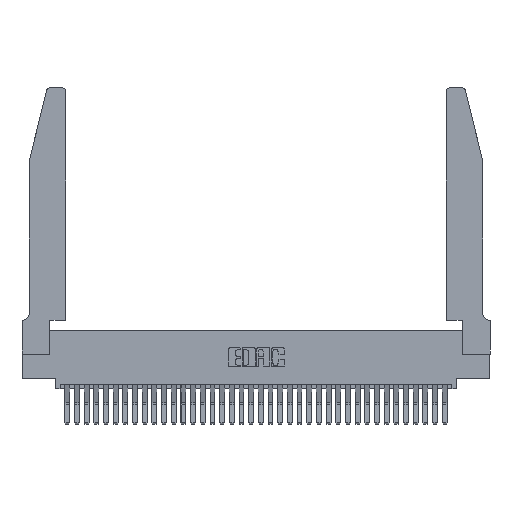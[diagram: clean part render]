
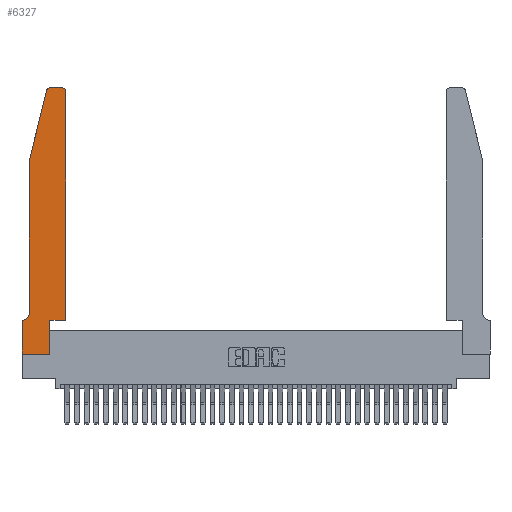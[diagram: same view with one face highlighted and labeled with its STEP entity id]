
A CAD part, top view. The second image highlights one B-rep face of the part: STEP entity #6327.
In plain terms, the highlighted planar face has unit normal (0, 0, 1).
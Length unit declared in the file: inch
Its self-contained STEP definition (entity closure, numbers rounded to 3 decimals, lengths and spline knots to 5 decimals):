
#99 = LINE ( 'NONE', #27117, #14691 ) ;
#202 = DIRECTION ( 'NONE',  ( -1., 0., 0. ) ) ;
#450 = CARTESIAN_POINT ( 'NONE',  ( 0.4205, 2.72, 0.37 ) ) ;
#1453 = DIRECTION ( 'NONE',  ( 0., 1., 0. ) ) ;
#1481 = ORIENTED_EDGE ( 'NONE', *, *, #2511, .T. ) ;
#1762 = CARTESIAN_POINT ( 'NONE',  ( 0.2605, 2.75, 0.37 ) ) ;
#2511 = EDGE_CURVE ( 'NONE', #35598, #21284, #27533, .T. ) ;
#2516 = VERTEX_POINT ( 'NONE', #13177 ) ;
#2844 = AXIS2_PLACEMENT_3D ( 'NONE', #29377, #12700, #32178 ) ;
#3141 = VECTOR ( 'NONE', #26268, 39.37008 ) ;
#3402 = DIRECTION ( 'NONE',  ( 1., 0., 0. ) ) ;
#3568 = CARTESIAN_POINT ( 'NONE',  ( 0.0755, 0.35, 0.37 ) ) ;
#3908 = CARTESIAN_POINT ( 'NONE',  ( 0.284, 2.75, 0.37 ) ) ;
#4074 = ORIENTED_EDGE ( 'NONE', *, *, #31906, .T. ) ;
#4113 = ORIENTED_EDGE ( 'NONE', *, *, #31915, .T. ) ;
#4151 = ORIENTED_EDGE ( 'NONE', *, *, #13359, .T. ) ;
#4364 = VERTEX_POINT ( 'NONE', #22695 ) ;
#4402 = CARTESIAN_POINT ( 'NONE',  ( 0.2865, 0.35, 0.37 ) ) ;
#4698 = CARTESIAN_POINT ( 'NONE',  ( 0., 0., 0.37 ) ) ;
#4884 = VERTEX_POINT ( 'NONE', #19773 ) ;
#4965 = VECTOR ( 'NONE', #1453, 39.37008 ) ;
#5477 = PLANE ( 'NONE',  #13334 ) ;
#5591 = DIRECTION ( 'NONE',  ( 1., 0., 0. ) ) ;
#6061 = EDGE_CURVE ( 'NONE', #27158, #4364, #34232, .T. ) ;
#6327 = ADVANCED_FACE ( 'NONE', ( #26391 ), #5477, .T. ) ;
#6561 = LINE ( 'NONE', #23788, #27309 ) ;
#6644 = EDGE_CURVE ( 'NONE', #10097, #32319, #24177, .T. ) ;
#7117 = CARTESIAN_POINT ( 'NONE',  ( 0., 0., 0.37 ) ) ;
#7408 = DIRECTION ( 'NONE',  ( 0., -1., 0. ) ) ;
#7522 = DIRECTION ( 'NONE',  ( -1., 0., 0. ) ) ;
#7606 = EDGE_LOOP ( 'NONE', ( #29742, #34257, #24436, #26052, #4074, #9270, #14604, #16992, #1481, #4113, #4151, #17957 ) ) ;
#7852 = CIRCLE ( 'NONE', #8065, 0.07 ) ;
#8065 = AXIS2_PLACEMENT_3D ( 'NONE', #34139, #17550, #202 ) ;
#8602 = AXIS2_PLACEMENT_3D ( 'NONE', #450, #20549, #3402 ) ;
#8672 = CIRCLE ( 'NONE', #8602, 0.03 ) ;
#8950 = VECTOR ( 'NONE', #27343, 39.37008 ) ;
#9270 = ORIENTED_EDGE ( 'NONE', *, *, #16638, .T. ) ;
#9965 = EDGE_CURVE ( 'NONE', #4884, #2516, #8672, .T. ) ;
#10097 = VERTEX_POINT ( 'NONE', #3908 ) ;
#11513 = CARTESIAN_POINT ( 'NONE',  ( 0.0755, 0.42, 0.37 ) ) ;
#11669 = EDGE_CURVE ( 'NONE', #2516, #10097, #36123, .T. ) ;
#12108 = CARTESIAN_POINT ( 'NONE',  ( 0.0755, 2., 0.37 ) ) ;
#12646 = CARTESIAN_POINT ( 'NONE',  ( 0.0755, 2., 0.37 ) ) ;
#12700 = DIRECTION ( 'NONE',  ( 0., 0., 1. ) ) ;
#13177 = CARTESIAN_POINT ( 'NONE',  ( 0.4205, 2.75, 0.37 ) ) ;
#13334 = AXIS2_PLACEMENT_3D ( 'NONE', #17090, #22622, #5591 ) ;
#13359 = EDGE_CURVE ( 'NONE', #24913, #4884, #6561, .T. ) ;
#13776 = CARTESIAN_POINT ( 'NONE',  ( 0.4505, 0.35, 0.37 ) ) ;
#14604 = ORIENTED_EDGE ( 'NONE', *, *, #6061, .T. ) ;
#14691 = VECTOR ( 'NONE', #7408, 39.37008 ) ;
#14724 = DIRECTION ( 'NONE',  ( 1., 0., 0. ) ) ;
#14790 = EDGE_CURVE ( 'NONE', #24642, #27037, #99, .T. ) ;
#14854 = VECTOR ( 'NONE', #7522, 39.37008 ) ;
#16638 = EDGE_CURVE ( 'NONE', #18704, #27158, #18467, .T. ) ;
#16992 = ORIENTED_EDGE ( 'NONE', *, *, #27493, .T. ) ;
#17090 = CARTESIAN_POINT ( 'NONE',  ( 0., 0.35, 0.37 ) ) ;
#17550 = DIRECTION ( 'NONE',  ( 0., 0., -1. ) ) ;
#17957 = ORIENTED_EDGE ( 'NONE', *, *, #9965, .T. ) ;
#18467 = LINE ( 'NONE', #3568, #3141 ) ;
#18704 = VERTEX_POINT ( 'NONE', #28279 ) ;
#19773 = CARTESIAN_POINT ( 'NONE',  ( 0.4505, 2.72, 0.37 ) ) ;
#20549 = DIRECTION ( 'NONE',  ( 0., 0., 1. ) ) ;
#21284 = VERTEX_POINT ( 'NONE', #22492 ) ;
#22060 = VECTOR ( 'NONE', #34887, 39.37008 ) ;
#22492 = CARTESIAN_POINT ( 'NONE',  ( 0.2865, 0.35, 0.37 ) ) ;
#22622 = DIRECTION ( 'NONE',  ( 0., 0., 1. ) ) ;
#22695 = CARTESIAN_POINT ( 'NONE',  ( 0., 0., 0.37 ) ) ;
#23493 = CARTESIAN_POINT ( 'NONE',  ( 0.2865, 0., 0.37 ) ) ;
#23788 = CARTESIAN_POINT ( 'NONE',  ( 0.4505, 0.35, 0.37 ) ) ;
#24177 = CIRCLE ( 'NONE', #2844, 0.03 ) ;
#24436 = ORIENTED_EDGE ( 'NONE', *, *, #31425, .T. ) ;
#24631 = LINE ( 'NONE', #12108, #22060 ) ;
#24642 = VERTEX_POINT ( 'NONE', #12646 ) ;
#24913 = VERTEX_POINT ( 'NONE', #13776 ) ;
#26052 = ORIENTED_EDGE ( 'NONE', *, *, #14790, .T. ) ;
#26268 = DIRECTION ( 'NONE',  ( -1., 0., 0. ) ) ;
#26391 = FACE_OUTER_BOUND ( 'NONE', #7606, .T. ) ;
#26604 = DIRECTION ( 'NONE',  ( 0., 1., 0. ) ) ;
#26848 = VECTOR ( 'NONE', #32432, 39.37008 ) ;
#27037 = VERTEX_POINT ( 'NONE', #11513 ) ;
#27117 = CARTESIAN_POINT ( 'NONE',  ( 0.0755, 2., 0.37 ) ) ;
#27158 = VERTEX_POINT ( 'NONE', #34287 ) ;
#27309 = VECTOR ( 'NONE', #26604, 39.37008 ) ;
#27343 = DIRECTION ( 'NONE',  ( 1., 0., 0. ) ) ;
#27493 = EDGE_CURVE ( 'NONE', #4364, #35598, #31301, .T. ) ;
#27533 = LINE ( 'NONE', #4402, #4965 ) ;
#28279 = CARTESIAN_POINT ( 'NONE',  ( 0.0055, 0.35, 0.37 ) ) ;
#28519 = VECTOR ( 'NONE', #14724, 39.37008 ) ;
#29377 = CARTESIAN_POINT ( 'NONE',  ( 0.284, 2.72, 0.37 ) ) ;
#29742 = ORIENTED_EDGE ( 'NONE', *, *, #11669, .T. ) ;
#30695 = CARTESIAN_POINT ( 'NONE',  ( 0.25487, 2.72718, 0.37 ) ) ;
#31301 = LINE ( 'NONE', #4698, #8950 ) ;
#31333 = CARTESIAN_POINT ( 'NONE',  ( 0.4505, 0.35, 0.37 ) ) ;
#31425 = EDGE_CURVE ( 'NONE', #32319, #24642, #24631, .T. ) ;
#31906 = EDGE_CURVE ( 'NONE', #27037, #18704, #7852, .T. ) ;
#31915 = EDGE_CURVE ( 'NONE', #21284, #24913, #35909, .T. ) ;
#32178 = DIRECTION ( 'NONE',  ( 1., 0., 0. ) ) ;
#32319 = VERTEX_POINT ( 'NONE', #30695 ) ;
#32432 = DIRECTION ( 'NONE',  ( 0., -1., 0. ) ) ;
#34139 = CARTESIAN_POINT ( 'NONE',  ( 0.0055, 0.42, 0.37 ) ) ;
#34232 = LINE ( 'NONE', #7117, #26848 ) ;
#34257 = ORIENTED_EDGE ( 'NONE', *, *, #6644, .T. ) ;
#34287 = CARTESIAN_POINT ( 'NONE',  ( 0., 0.35, 0.37 ) ) ;
#34887 = DIRECTION ( 'NONE',  ( -0.239, -0.971, 0. ) ) ;
#35598 = VERTEX_POINT ( 'NONE', #23493 ) ;
#35909 = LINE ( 'NONE', #31333, #28519 ) ;
#36123 = LINE ( 'NONE', #1762, #14854 ) ;
